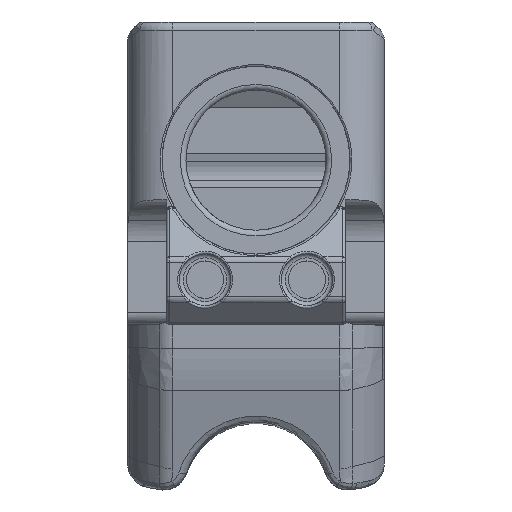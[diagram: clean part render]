
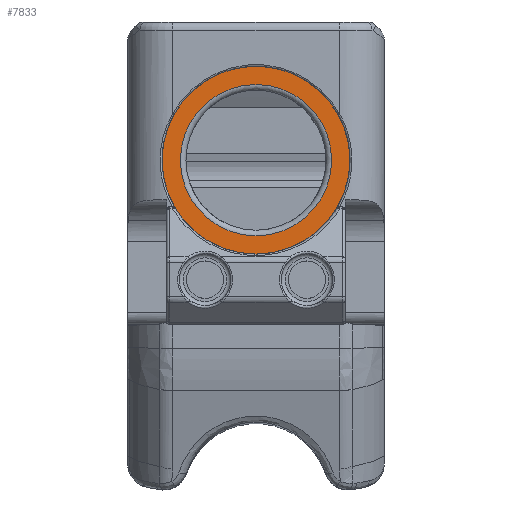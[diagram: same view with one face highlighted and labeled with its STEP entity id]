
A CAD part, front view. The second image highlights one B-rep face of the part: STEP entity #7833.
In plain terms, the highlighted planar face has unit normal (0, -1, 0).
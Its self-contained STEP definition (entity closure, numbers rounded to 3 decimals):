
#72=FACE_BOUND('',#2099,.T.);
#192=PLANE('',#8368);
#1598=FACE_OUTER_BOUND('',#2098,.T.);
#2098=EDGE_LOOP('',(#5442));
#2099=EDGE_LOOP('',(#5443));
#2591=CIRCLE('',#8330,9.425);
#2600=CIRCLE('',#8369,11.697);
#3278=VERTEX_POINT('',#11957);
#3341=VERTEX_POINT('',#12531);
#4036=EDGE_CURVE('',#3278,#3278,#2591,.T.);
#4127=EDGE_CURVE('',#3341,#3341,#2600,.T.);
#5442=ORIENTED_EDGE('',*,*,#4127,.T.);
#5443=ORIENTED_EDGE('',*,*,#4036,.F.);
#7833=ADVANCED_FACE('',(#1598,#72),#192,.T.);
#8330=AXIS2_PLACEMENT_3D('',#11958,#9268,#9269);
#8368=AXIS2_PLACEMENT_3D('',#12530,#9394,#9395);
#8369=AXIS2_PLACEMENT_3D('',#12532,#9396,#9397);
#9268=DIRECTION('center_axis',(0.,-1.,0.));
#9269=DIRECTION('ref_axis',(0.922,0.,0.388));
#9394=DIRECTION('center_axis',(0.,-1.,0.));
#9395=DIRECTION('ref_axis',(1.,0.,0.));
#9396=DIRECTION('center_axis',(0.,-1.,0.));
#9397=DIRECTION('ref_axis',(1.,0.,0.));
#11957=CARTESIAN_POINT('',(15.977,-18.733,-125.541));
#11958=CARTESIAN_POINT('Origin',(15.977,-18.733,-116.116));
#12530=CARTESIAN_POINT('Origin',(15.977,-18.733,-116.116));
#12531=CARTESIAN_POINT('',(15.977,-18.733,-127.813));
#12532=CARTESIAN_POINT('Origin',(15.977,-18.733,-116.116));
